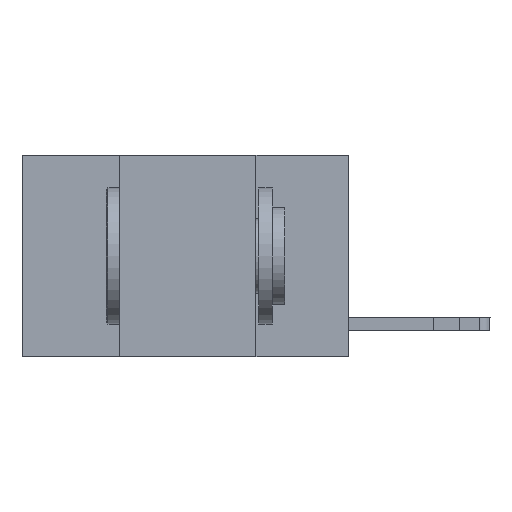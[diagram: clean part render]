
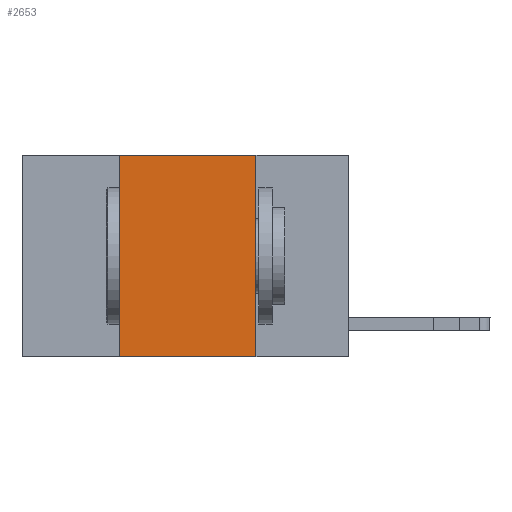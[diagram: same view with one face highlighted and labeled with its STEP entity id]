
A CAD part, left-side view. The second image highlights one B-rep face of the part: STEP entity #2653.
In plain terms, the highlighted planar face has unit normal (-1, 0, 0).
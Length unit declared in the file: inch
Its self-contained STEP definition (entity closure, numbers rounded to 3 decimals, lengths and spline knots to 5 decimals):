
#566 = CARTESIAN_POINT ( 'NONE',  ( 0., 0.17, 0. ) ) ;
#1077 = EDGE_CURVE ( 'NONE', #5819, #7130, #5734, .T. ) ;
#1084 = VECTOR ( 'NONE', #17153, 39.37008 ) ;
#2041 = LINE ( 'NONE', #566, #2461 ) ;
#2461 = VECTOR ( 'NONE', #4662, 39.37008 ) ;
#2530 = ORIENTED_EDGE ( 'NONE', *, *, #4961, .F. ) ;
#2549 = ORIENTED_EDGE ( 'NONE', *, *, #4472, .F. ) ;
#2653 = ADVANCED_FACE ( 'NONE', ( #10477 ), #11862, .F. ) ;
#3362 = DIRECTION ( 'NONE',  ( 0., 0., -1. ) ) ;
#4472 = EDGE_CURVE ( 'NONE', #16762, #16300, #13714, .T. ) ;
#4662 = DIRECTION ( 'NONE',  ( 0., 0., -1. ) ) ;
#4916 = EDGE_LOOP ( 'NONE', ( #9141, #2549, #2530, #13323 ) ) ;
#4961 = EDGE_CURVE ( 'NONE', #5819, #16762, #15482, .T. ) ;
#5130 = CARTESIAN_POINT ( 'NONE',  ( 0., 0.6, 0. ) ) ;
#5734 = LINE ( 'NONE', #11423, #1084 ) ;
#5819 = VERTEX_POINT ( 'NONE', #15341 ) ;
#7130 = VERTEX_POINT ( 'NONE', #10164 ) ;
#9141 = ORIENTED_EDGE ( 'NONE', *, *, #16249, .F. ) ;
#9272 = DIRECTION ( 'NONE',  ( 1., 0., 0. ) ) ;
#9820 = DIRECTION ( 'NONE',  ( 0., -1., 0. ) ) ;
#9903 = CARTESIAN_POINT ( 'NONE',  ( 0., 0.6, 0. ) ) ;
#10164 = CARTESIAN_POINT ( 'NONE',  ( 0., 0.17, -0.37 ) ) ;
#10477 = FACE_OUTER_BOUND ( 'NONE', #4916, .T. ) ;
#11423 = CARTESIAN_POINT ( 'NONE',  ( 0., 0.6, -0.37 ) ) ;
#11862 = PLANE ( 'NONE',  #13529 ) ;
#12912 = CARTESIAN_POINT ( 'NONE',  ( 0., 0.17, 0. ) ) ;
#13323 = ORIENTED_EDGE ( 'NONE', *, *, #1077, .T. ) ;
#13493 = VECTOR ( 'NONE', #16710, 39.37008 ) ;
#13529 = AXIS2_PLACEMENT_3D ( 'NONE', #5130, #9272, #3362 ) ;
#13714 = LINE ( 'NONE', #9903, #16475 ) ;
#15341 = CARTESIAN_POINT ( 'NONE',  ( 0., 0.42, -0.37 ) ) ;
#15482 = LINE ( 'NONE', #16893, #13493 ) ;
#16249 = EDGE_CURVE ( 'NONE', #16300, #7130, #2041, .T. ) ;
#16300 = VERTEX_POINT ( 'NONE', #12912 ) ;
#16475 = VECTOR ( 'NONE', #9820, 39.37008 ) ;
#16710 = DIRECTION ( 'NONE',  ( 0., 0., 1. ) ) ;
#16762 = VERTEX_POINT ( 'NONE', #17921 ) ;
#16893 = CARTESIAN_POINT ( 'NONE',  ( 0., 0.42, 0. ) ) ;
#17153 = DIRECTION ( 'NONE',  ( 0., -1., 0. ) ) ;
#17921 = CARTESIAN_POINT ( 'NONE',  ( 0., 0.42, 0. ) ) ;
